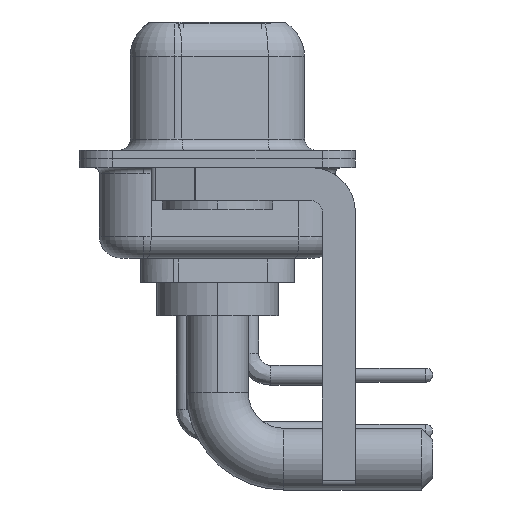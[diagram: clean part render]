
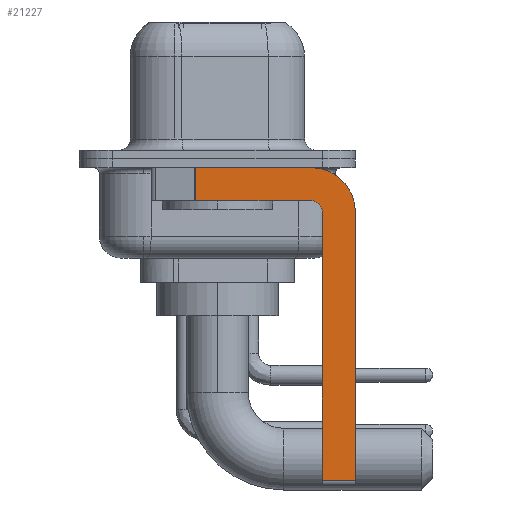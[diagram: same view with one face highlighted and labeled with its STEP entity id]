
A CAD part, left-side view. The second image highlights one B-rep face of the part: STEP entity #21227.
In plain terms, the highlighted planar face has unit normal (-1, 0, 0).
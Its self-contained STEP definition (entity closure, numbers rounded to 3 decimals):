
#514 = EDGE_CURVE ( 'NONE', #23781, #22459, #6220, .T. ) ;
#533 = CARTESIAN_POINT ( 'NONE',  ( -2.9, -4.25, -14.55 ) ) ;
#580 = VERTEX_POINT ( 'NONE', #21268 ) ;
#652 = LINE ( 'NONE', #4031, #19262 ) ;
#1273 = VERTEX_POINT ( 'NONE', #1576 ) ;
#1415 = EDGE_LOOP ( 'NONE', ( #17463, #5995, #18849, #11394, #5194, #3656, #12826, #7496 ) ) ;
#1576 = CARTESIAN_POINT ( 'NONE',  ( -2.9, -4.25, -1.9 ) ) ;
#1799 = DIRECTION ( 'NONE',  ( 1., 0., 0. ) ) ;
#1837 = CARTESIAN_POINT ( 'NONE',  ( -2.9, -4.75, -2.4 ) ) ;
#2761 = CARTESIAN_POINT ( 'NONE',  ( -2.9, -4.75, -14.8 ) ) ;
#3656 = ORIENTED_EDGE ( 'NONE', *, *, #8195, .T. ) ;
#4031 = CARTESIAN_POINT ( 'NONE',  ( -2.9, 0.978, -1.9 ) ) ;
#4340 = DIRECTION ( 'NONE',  ( 0., -1., 0. ) ) ;
#4703 = LINE ( 'NONE', #23226, #13145 ) ;
#5194 = ORIENTED_EDGE ( 'NONE', *, *, #6029, .F. ) ;
#5607 = DIRECTION ( 'NONE',  ( -1., 0., 0. ) ) ;
#5995 = ORIENTED_EDGE ( 'NONE', *, *, #8264, .T. ) ;
#6005 = DIRECTION ( 'NONE',  ( 0., 0., -1. ) ) ;
#6029 = EDGE_CURVE ( 'NONE', #20723, #11593, #8608, .T. ) ;
#6131 = CARTESIAN_POINT ( 'NONE',  ( -2.9, -6.25, -2.4 ) ) ;
#6220 = LINE ( 'NONE', #13815, #24449 ) ;
#6677 = VERTEX_POINT ( 'NONE', #16420 ) ;
#7140 = EDGE_CURVE ( 'NONE', #1273, #580, #8555, .T. ) ;
#7496 = ORIENTED_EDGE ( 'NONE', *, *, #17972, .F. ) ;
#8195 = EDGE_CURVE ( 'NONE', #20723, #22459, #21543, .T. ) ;
#8264 = EDGE_CURVE ( 'NONE', #6677, #580, #652, .T. ) ;
#8555 = LINE ( 'NONE', #18367, #10390 ) ;
#8608 = LINE ( 'NONE', #2761, #23956 ) ;
#9512 = PLANE ( 'NONE',  #20955 ) ;
#10122 = DIRECTION ( 'NONE',  ( 0., -1., 0. ) ) ;
#10390 = VECTOR ( 'NONE', #21843, 1000. ) ;
#10421 = VERTEX_POINT ( 'NONE', #22968 ) ;
#10663 = CIRCLE ( 'NONE', #18202, 0.5 ) ;
#11394 = ORIENTED_EDGE ( 'NONE', *, *, #21506, .F. ) ;
#11593 = VERTEX_POINT ( 'NONE', #1837 ) ;
#12826 = ORIENTED_EDGE ( 'NONE', *, *, #514, .F. ) ;
#13145 = VECTOR ( 'NONE', #4340, 1000. ) ;
#13777 = EDGE_CURVE ( 'NONE', #6677, #10421, #4703, .T. ) ;
#13815 = CARTESIAN_POINT ( 'NONE',  ( -2.9, -6.25, -2.4 ) ) ;
#15833 = DIRECTION ( 'NONE',  ( 1., 0., 0. ) ) ;
#16085 = CARTESIAN_POINT ( 'NONE',  ( -2.9, -4.25, -2.4 ) ) ;
#16198 = DIRECTION ( 'NONE',  ( 0., 0., -1. ) ) ;
#16420 = CARTESIAN_POINT ( 'NONE',  ( -2.9, 0.978, -0.4 ) ) ;
#17096 = DIRECTION ( 'NONE',  ( 0., 0., -1. ) ) ;
#17463 = ORIENTED_EDGE ( 'NONE', *, *, #13777, .F. ) ;
#17972 = EDGE_CURVE ( 'NONE', #10421, #23781, #24357, .T. ) ;
#18172 = CARTESIAN_POINT ( 'NONE',  ( -2.9, -6.25, -14.55 ) ) ;
#18202 = AXIS2_PLACEMENT_3D ( 'NONE', #23995, #5607, #20517 ) ;
#18367 = CARTESIAN_POINT ( 'NONE',  ( -2.9, -4.25, -1.9 ) ) ;
#18849 = ORIENTED_EDGE ( 'NONE', *, *, #7140, .F. ) ;
#19262 = VECTOR ( 'NONE', #6005, 1000. ) ;
#19915 = DIRECTION ( 'NONE',  ( 0., 0., 1. ) ) ;
#20400 = AXIS2_PLACEMENT_3D ( 'NONE', #16085, #15833, #16198 ) ;
#20517 = DIRECTION ( 'NONE',  ( 0., 0., 1. ) ) ;
#20723 = VERTEX_POINT ( 'NONE', #22586 ) ;
#20955 = AXIS2_PLACEMENT_3D ( 'NONE', #24531, #1799, #17096 ) ;
#21227 = ADVANCED_FACE ( 'NONE', ( #22558 ), #9512, .F. ) ;
#21268 = CARTESIAN_POINT ( 'NONE',  ( -2.9, 0.978, -1.9 ) ) ;
#21506 = EDGE_CURVE ( 'NONE', #11593, #1273, #10663, .T. ) ;
#21513 = DIRECTION ( 'NONE',  ( 0., 0., -1. ) ) ;
#21543 = LINE ( 'NONE', #533, #22812 ) ;
#21843 = DIRECTION ( 'NONE',  ( 0., 1., 0. ) ) ;
#22459 = VERTEX_POINT ( 'NONE', #18172 ) ;
#22558 = FACE_OUTER_BOUND ( 'NONE', #1415, .T. ) ;
#22586 = CARTESIAN_POINT ( 'NONE',  ( -2.9, -4.75, -14.55 ) ) ;
#22812 = VECTOR ( 'NONE', #10122, 1000. ) ;
#22968 = CARTESIAN_POINT ( 'NONE',  ( -2.9, -4.25, -0.4 ) ) ;
#23226 = CARTESIAN_POINT ( 'NONE',  ( -2.9, 3., -0.4 ) ) ;
#23781 = VERTEX_POINT ( 'NONE', #6131 ) ;
#23956 = VECTOR ( 'NONE', #19915, 1000. ) ;
#23995 = CARTESIAN_POINT ( 'NONE',  ( -2.9, -4.25, -2.4 ) ) ;
#24357 = CIRCLE ( 'NONE', #20400, 2. ) ;
#24449 = VECTOR ( 'NONE', #21513, 1000. ) ;
#24531 = CARTESIAN_POINT ( 'NONE',  ( -2.9, -4.25, -2.4 ) ) ;
